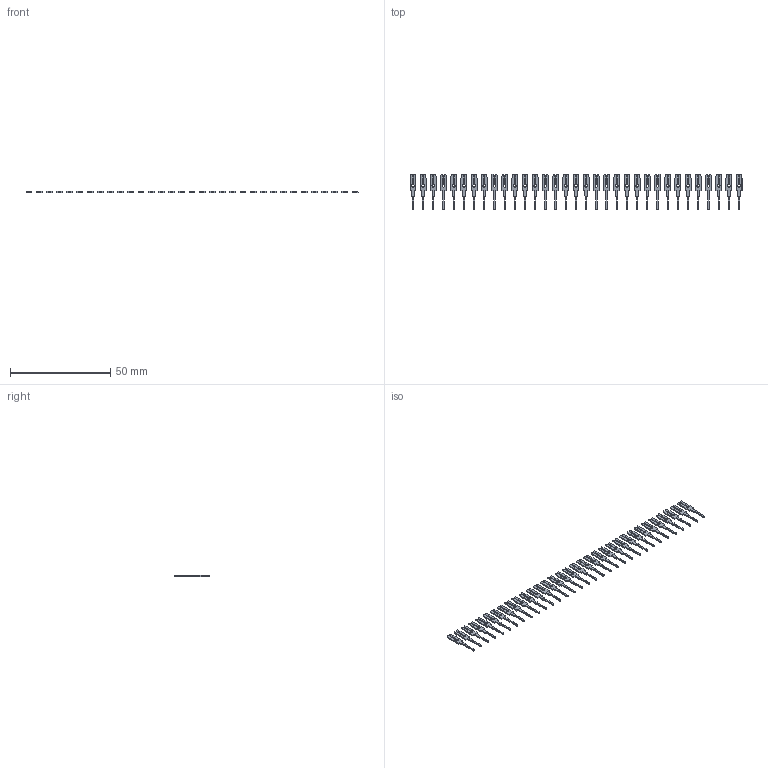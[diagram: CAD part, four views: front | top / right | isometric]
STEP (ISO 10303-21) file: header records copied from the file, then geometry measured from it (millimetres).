
FILE_DESCRIPTION (( 'STEP AP203' ), '1' );
FILE_NAME ('103-033-251-200.STEP', '2020-04-09T20:57:51', ( '' ), ( '' ), 'SwSTEP 2.0', 'SolidWorks 2016', '' );
FILE_SCHEMA (( 'CONFIG_CONTROL_DESIGN' ));
Length unit declared in the file: inch
Products named in the file (2): 103-033-251-200; 100-290-001_100-290-251
Assembly tree (33 placements, depth 2):
  103-033-251-200
    100-290-001_100-290-251  x33
Bounding box: 165.48 x 17.91 x 0.66 mm (x, y, z)
Volume: 603.4 mm3; surface area: 2965.6 mm2
Topology: 33 solids, 33 shells, 924 faces, 2574 edges, 1716 vertices
Faces by surface type: plane 726, cylinder 198
Entity records: 2118 total; most frequent: DIRECTION 214, CARTESIAN_POINT 206, ORIENTED_EDGE 156, EDGE_CURVE 78, LOCAL_TIME 76, CALENDAR_DATE 76, AXIS2_PLACEMENT_3D 76, COORDINATED_UNIVERSAL_TIME_OFFSET 76
